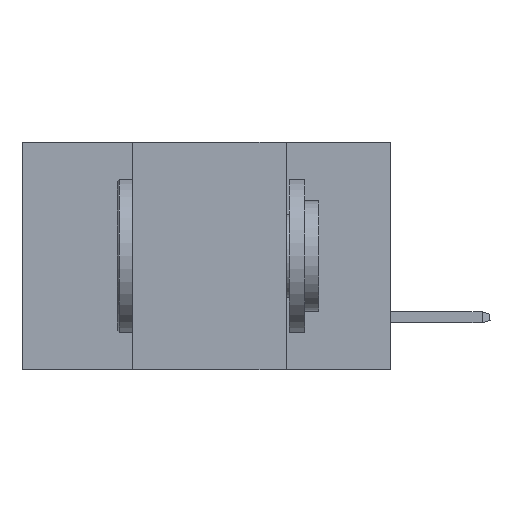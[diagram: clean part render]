
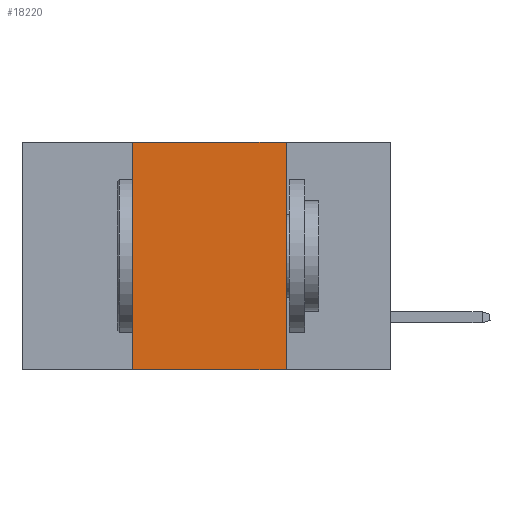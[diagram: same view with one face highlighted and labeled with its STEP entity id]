
A CAD part, left-side view. The second image highlights one B-rep face of the part: STEP entity #18220.
In plain terms, the highlighted planar face has unit normal (-1, 0, 0).
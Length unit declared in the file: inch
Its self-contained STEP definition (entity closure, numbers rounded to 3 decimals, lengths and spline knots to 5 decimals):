
#815 = ORIENTED_EDGE ( 'NONE', *, *, #2508, .T. ) ;
#1411 = CARTESIAN_POINT ( 'NONE',  ( 0., 0.6, -0.37 ) ) ;
#1425 = EDGE_CURVE ( 'NONE', #24861, #19588, #22928, .T. ) ;
#2258 = DIRECTION ( 'NONE',  ( 0., 0., -1. ) ) ;
#2508 = EDGE_CURVE ( 'NONE', #23635, #3047, #8884, .T. ) ;
#2513 = VECTOR ( 'NONE', #20304, 39.37008 ) ;
#2874 = VECTOR ( 'NONE', #25347, 39.37008 ) ;
#3047 = VERTEX_POINT ( 'NONE', #11919 ) ;
#4333 = ORIENTED_EDGE ( 'NONE', *, *, #20429, .F. ) ;
#6540 = CARTESIAN_POINT ( 'NONE',  ( 0., 0.42, 0. ) ) ;
#6760 = CARTESIAN_POINT ( 'NONE',  ( 0., 0.6, 0. ) ) ;
#7052 = DIRECTION ( 'NONE',  ( 0., 0., -1. ) ) ;
#8342 = ORIENTED_EDGE ( 'NONE', *, *, #26715, .F. ) ;
#8884 = LINE ( 'NONE', #1411, #2513 ) ;
#10268 = VECTOR ( 'NONE', #20864, 39.37008 ) ;
#11261 = PLANE ( 'NONE',  #17405 ) ;
#11919 = CARTESIAN_POINT ( 'NONE',  ( 0., 0.17, -0.37 ) ) ;
#12949 = ORIENTED_EDGE ( 'NONE', *, *, #1425, .F. ) ;
#13038 = EDGE_LOOP ( 'NONE', ( #8342, #12949, #4333, #815 ) ) ;
#13045 = CARTESIAN_POINT ( 'NONE',  ( 0., 0.17, 0. ) ) ;
#13067 = CARTESIAN_POINT ( 'NONE',  ( 0., 0.42, -0.37 ) ) ;
#13786 = CARTESIAN_POINT ( 'NONE',  ( 0., 0.6, 0. ) ) ;
#17405 = AXIS2_PLACEMENT_3D ( 'NONE', #6760, #18559, #2258 ) ;
#17622 = LINE ( 'NONE', #13045, #25043 ) ;
#18220 = ADVANCED_FACE ( 'NONE', ( #27787 ), #11261, .F. ) ;
#18559 = DIRECTION ( 'NONE',  ( 1., 0., 0. ) ) ;
#19588 = VERTEX_POINT ( 'NONE', #21799 ) ;
#20304 = DIRECTION ( 'NONE',  ( 0., -1., 0. ) ) ;
#20429 = EDGE_CURVE ( 'NONE', #23635, #24861, #25438, .T. ) ;
#20864 = DIRECTION ( 'NONE',  ( 0., 0., 1. ) ) ;
#21799 = CARTESIAN_POINT ( 'NONE',  ( 0., 0.17, 0. ) ) ;
#22928 = LINE ( 'NONE', #13786, #2874 ) ;
#23635 = VERTEX_POINT ( 'NONE', #13067 ) ;
#24861 = VERTEX_POINT ( 'NONE', #28161 ) ;
#25043 = VECTOR ( 'NONE', #7052, 39.37008 ) ;
#25347 = DIRECTION ( 'NONE',  ( 0., -1., 0. ) ) ;
#25438 = LINE ( 'NONE', #6540, #10268 ) ;
#26715 = EDGE_CURVE ( 'NONE', #19588, #3047, #17622, .T. ) ;
#27787 = FACE_OUTER_BOUND ( 'NONE', #13038, .T. ) ;
#28161 = CARTESIAN_POINT ( 'NONE',  ( 0., 0.42, 0. ) ) ;
